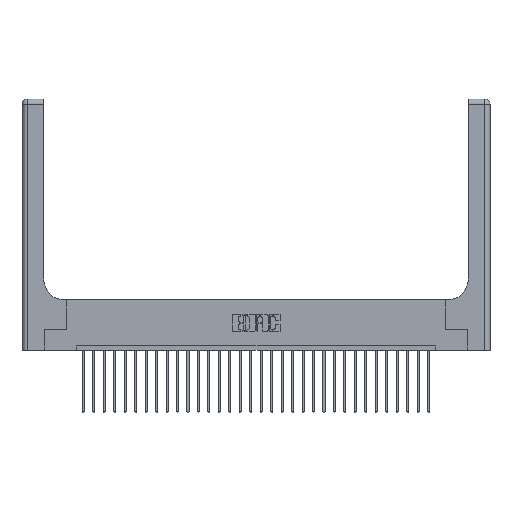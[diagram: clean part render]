
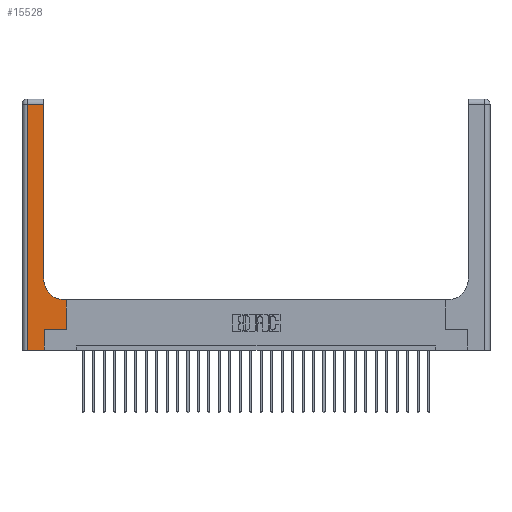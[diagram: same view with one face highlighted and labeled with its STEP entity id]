
A CAD part, top view. The second image highlights one B-rep face of the part: STEP entity #15528.
In plain terms, the highlighted planar face has unit normal (0, 0, 1).
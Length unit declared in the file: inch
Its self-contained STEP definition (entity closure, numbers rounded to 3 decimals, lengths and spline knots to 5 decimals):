
#104 = EDGE_CURVE ( 'NONE', #8241, #19850, #5252, .T. ) ;
#451 = LINE ( 'NONE', #18024, #22324 ) ;
#720 = LINE ( 'NONE', #16800, #21807 ) ;
#836 = CARTESIAN_POINT ( 'NONE',  ( 0.265, 0.25, 0.37 ) ) ;
#961 = VERTEX_POINT ( 'NONE', #836 ) ;
#1142 = VECTOR ( 'NONE', #7597, 39.37008 ) ;
#1701 = CARTESIAN_POINT ( 'NONE',  ( 0.265, 0.25, 0.37 ) ) ;
#1995 = DIRECTION ( 'NONE',  ( 1., 0., 0. ) ) ;
#2324 = CARTESIAN_POINT ( 'NONE',  ( 0.06, 0., 0.37 ) ) ;
#2447 = DIRECTION ( 'NONE',  ( 0., 1., 0. ) ) ;
#3135 = CARTESIAN_POINT ( 'NONE',  ( 0.528, 0.25, 0.37 ) ) ;
#3625 = PLANE ( 'NONE',  #19364 ) ;
#3633 = VERTEX_POINT ( 'NONE', #3135 ) ;
#3814 = DIRECTION ( 'NONE',  ( 0., 0., -1. ) ) ;
#5101 = CARTESIAN_POINT ( 'NONE',  ( 0.265, 0., 0.37 ) ) ;
#5183 = CARTESIAN_POINT ( 'NONE',  ( 0.26, 0.85, 0.37 ) ) ;
#5252 = LINE ( 'NONE', #9621, #14587 ) ;
#5424 = CARTESIAN_POINT ( 'NONE',  ( 0.06, 3., 0.37 ) ) ;
#5624 = EDGE_CURVE ( 'NONE', #961, #3633, #9717, .T. ) ;
#5839 = LINE ( 'NONE', #7798, #14886 ) ;
#6369 = ORIENTED_EDGE ( 'NONE', *, *, #5624, .T. ) ;
#6550 = EDGE_CURVE ( 'NONE', #10001, #18878, #10539, .T. ) ;
#6655 = ORIENTED_EDGE ( 'NONE', *, *, #6550, .T. ) ;
#6720 = CARTESIAN_POINT ( 'NONE',  ( 0.06, 2.94, 0.37 ) ) ;
#7223 = ORIENTED_EDGE ( 'NONE', *, *, #16167, .T. ) ;
#7464 = EDGE_CURVE ( 'NONE', #27789, #10875, #720, .T. ) ;
#7505 = EDGE_LOOP ( 'NONE', ( #25937, #9820, #9541, #6655, #7223, #6369, #13327, #17340, #27142 ) ) ;
#7509 = VECTOR ( 'NONE', #7806, 39.37008 ) ;
#7517 = DIRECTION ( 'NONE',  ( 0., 1., 0. ) ) ;
#7597 = DIRECTION ( 'NONE',  ( 1., 0., 0. ) ) ;
#7798 = CARTESIAN_POINT ( 'NONE',  ( 0.26, 3., 0.37 ) ) ;
#7806 = DIRECTION ( 'NONE',  ( 0., -1., 0. ) ) ;
#8241 = VERTEX_POINT ( 'NONE', #21341 ) ;
#9157 = EDGE_CURVE ( 'NONE', #3633, #27789, #451, .T. ) ;
#9541 = ORIENTED_EDGE ( 'NONE', *, *, #9797, .T. ) ;
#9621 = CARTESIAN_POINT ( 'NONE',  ( 0., 2.94, 0.37 ) ) ;
#9717 = LINE ( 'NONE', #1701, #1142 ) ;
#9797 = EDGE_CURVE ( 'NONE', #19850, #10001, #24705, .T. ) ;
#9820 = ORIENTED_EDGE ( 'NONE', *, *, #104, .T. ) ;
#10001 = VERTEX_POINT ( 'NONE', #2324 ) ;
#10087 = CARTESIAN_POINT ( 'NONE',  ( 0., 3., 0.37 ) ) ;
#10403 = CARTESIAN_POINT ( 'NONE',  ( 0., 0., 0.37 ) ) ;
#10539 = LINE ( 'NONE', #10403, #26279 ) ;
#10875 = VERTEX_POINT ( 'NONE', #15177 ) ;
#11277 = DIRECTION ( 'NONE',  ( 0., 1., 0. ) ) ;
#12448 = VERTEX_POINT ( 'NONE', #5183 ) ;
#13259 = CARTESIAN_POINT ( 'NONE',  ( 0.528, 0.6, 0.37 ) ) ;
#13327 = ORIENTED_EDGE ( 'NONE', *, *, #9157, .T. ) ;
#13440 = EDGE_CURVE ( 'NONE', #10875, #12448, #25140, .T. ) ;
#14587 = VECTOR ( 'NONE', #22842, 39.37008 ) ;
#14886 = VECTOR ( 'NONE', #7517, 39.37008 ) ;
#15177 = CARTESIAN_POINT ( 'NONE',  ( 0.51, 0.6, 0.37 ) ) ;
#15528 = ADVANCED_FACE ( 'NONE', ( #22610 ), #3625, .F. ) ;
#15982 = EDGE_CURVE ( 'NONE', #12448, #8241, #5839, .T. ) ;
#16126 = CARTESIAN_POINT ( 'NONE',  ( 0.265, 0., 0.37 ) ) ;
#16167 = EDGE_CURVE ( 'NONE', #18878, #961, #23963, .T. ) ;
#16800 = CARTESIAN_POINT ( 'NONE',  ( 0.26, 0.6, 0.37 ) ) ;
#17340 = ORIENTED_EDGE ( 'NONE', *, *, #7464, .T. ) ;
#17941 = AXIS2_PLACEMENT_3D ( 'NONE', #21250, #3814, #1995 ) ;
#18024 = CARTESIAN_POINT ( 'NONE',  ( 0.528, 0.25, 0.37 ) ) ;
#18878 = VERTEX_POINT ( 'NONE', #16126 ) ;
#19364 = AXIS2_PLACEMENT_3D ( 'NONE', #10087, #24870, #27126 ) ;
#19850 = VERTEX_POINT ( 'NONE', #6720 ) ;
#21164 = DIRECTION ( 'NONE',  ( -1., 0., 0. ) ) ;
#21250 = CARTESIAN_POINT ( 'NONE',  ( 0.51, 0.85, 0.37 ) ) ;
#21341 = CARTESIAN_POINT ( 'NONE',  ( 0.26, 2.94, 0.37 ) ) ;
#21807 = VECTOR ( 'NONE', #21164, 39.37008 ) ;
#22324 = VECTOR ( 'NONE', #11277, 39.37008 ) ;
#22610 = FACE_OUTER_BOUND ( 'NONE', #7505, .T. ) ;
#22842 = DIRECTION ( 'NONE',  ( -1., 0., 0. ) ) ;
#22991 = VECTOR ( 'NONE', #2447, 39.37008 ) ;
#23963 = LINE ( 'NONE', #5101, #22991 ) ;
#24705 = LINE ( 'NONE', #5424, #7509 ) ;
#24870 = DIRECTION ( 'NONE',  ( 0., 0., -1. ) ) ;
#25140 = CIRCLE ( 'NONE', #17941, 0.25 ) ;
#25937 = ORIENTED_EDGE ( 'NONE', *, *, #15982, .T. ) ;
#26279 = VECTOR ( 'NONE', #27577, 39.37008 ) ;
#27126 = DIRECTION ( 'NONE',  ( -1., 0., 0. ) ) ;
#27142 = ORIENTED_EDGE ( 'NONE', *, *, #13440, .T. ) ;
#27577 = DIRECTION ( 'NONE',  ( 1., 0., 0. ) ) ;
#27789 = VERTEX_POINT ( 'NONE', #13259 ) ;
